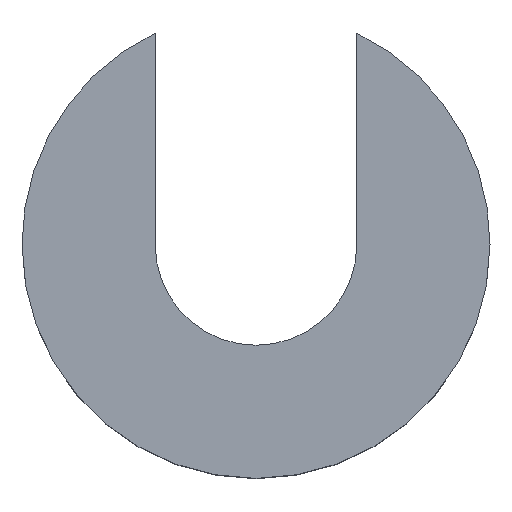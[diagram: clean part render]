
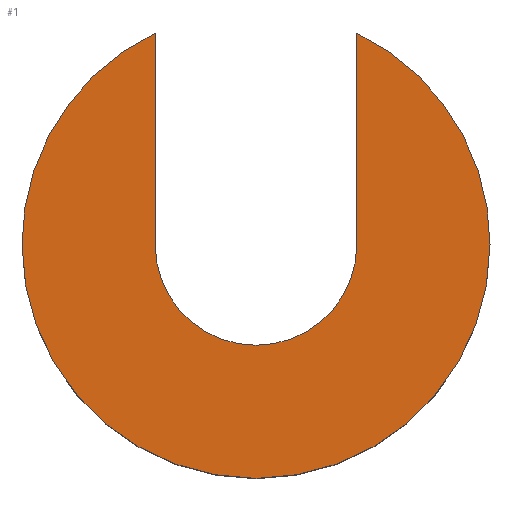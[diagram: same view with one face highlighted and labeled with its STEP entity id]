
A CAD part, top view. The second image highlights one B-rep face of the part: STEP entity #1.
In plain terms, the highlighted planar face has unit normal (0, 0, 1).
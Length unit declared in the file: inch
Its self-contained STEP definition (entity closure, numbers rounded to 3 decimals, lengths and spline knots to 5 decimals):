
#1 = ADVANCED_FACE ( 'NONE', ( #3 ), #357, .T. ) ;
#3 = FACE_OUTER_BOUND ( 'NONE', #412, .T. ) ;
#9 = DIRECTION ( 'NONE',  ( 1., 0., 0. ) ) ;
#15 = VECTOR ( 'NONE', #235, 39.37008 ) ;
#33 = CIRCLE ( 'NONE', #145, 0.725 ) ;
#46 = CARTESIAN_POINT ( 'NONE',  ( 0.3125, 0., 0.75 ) ) ;
#47 = CARTESIAN_POINT ( 'NONE',  ( -0.3125, 0., 0.75 ) ) ;
#73 = VECTOR ( 'NONE', #165, 39.37008 ) ;
#74 = EDGE_CURVE ( 'NONE', #184, #459, #276, .T. ) ;
#92 = EDGE_CURVE ( 'NONE', #459, #430, #388, .T. ) ;
#103 = DIRECTION ( 'NONE',  ( 0., 0., -1. ) ) ;
#118 = AXIS2_PLACEMENT_3D ( 'NONE', #179, #460, #325 ) ;
#119 = CARTESIAN_POINT ( 'NONE',  ( 0.725, 0., 0.75 ) ) ;
#123 = CIRCLE ( 'NONE', #170, 0.725 ) ;
#145 = AXIS2_PLACEMENT_3D ( 'NONE', #436, #271, #9 ) ;
#151 = EDGE_CURVE ( 'NONE', #400, #184, #166, .T. ) ;
#155 = CARTESIAN_POINT ( 'NONE',  ( 0., 0., 0.75 ) ) ;
#157 = CIRCLE ( 'NONE', #448, 0.725 ) ;
#165 = DIRECTION ( 'NONE',  ( 0., 1., 0. ) ) ;
#166 = LINE ( 'NONE', #201, #15 ) ;
#170 = AXIS2_PLACEMENT_3D ( 'NONE', #209, #349, #318 ) ;
#177 = EDGE_CURVE ( 'NONE', #368, #400, #33, .T. ) ;
#179 = CARTESIAN_POINT ( 'NONE',  ( 0., 0., 0.75 ) ) ;
#184 = VERTEX_POINT ( 'NONE', #46 ) ;
#201 = CARTESIAN_POINT ( 'NONE',  ( 0.3125, 0.65419, 0.75 ) ) ;
#204 = CARTESIAN_POINT ( 'NONE',  ( -0.3125, 0., 0.75 ) ) ;
#206 = EDGE_CURVE ( 'NONE', #430, #290, #123, .T. ) ;
#209 = CARTESIAN_POINT ( 'NONE',  ( 0., 0., 0.75 ) ) ;
#235 = DIRECTION ( 'NONE',  ( 0., -1., 0. ) ) ;
#237 = CARTESIAN_POINT ( 'NONE',  ( -0.3125, 0.65419, 0.75 ) ) ;
#271 = DIRECTION ( 'NONE',  ( 0., 0., 1. ) ) ;
#274 = ORIENTED_EDGE ( 'NONE', *, *, #151, .T. ) ;
#276 = CIRCLE ( 'NONE', #337, 0.3125 ) ;
#287 = DIRECTION ( 'NONE',  ( 1., 0., 0. ) ) ;
#290 = VERTEX_POINT ( 'NONE', #418 ) ;
#318 = DIRECTION ( 'NONE',  ( 1., 0., 0. ) ) ;
#325 = DIRECTION ( 'NONE',  ( 1., 0., 0. ) ) ;
#329 = ORIENTED_EDGE ( 'NONE', *, *, #177, .T. ) ;
#337 = AXIS2_PLACEMENT_3D ( 'NONE', #422, #103, #287 ) ;
#349 = DIRECTION ( 'NONE',  ( 0., 0., 1. ) ) ;
#357 = PLANE ( 'NONE',  #118 ) ;
#365 = ORIENTED_EDGE ( 'NONE', *, *, #369, .T. ) ;
#368 = VERTEX_POINT ( 'NONE', #119 ) ;
#369 = EDGE_CURVE ( 'NONE', #290, #368, #157, .T. ) ;
#378 = CARTESIAN_POINT ( 'NONE',  ( 0.3125, 0.65419, 0.75 ) ) ;
#388 = LINE ( 'NONE', #204, #73 ) ;
#395 = ORIENTED_EDGE ( 'NONE', *, *, #92, .T. ) ;
#400 = VERTEX_POINT ( 'NONE', #378 ) ;
#403 = DIRECTION ( 'NONE',  ( 0., 0., 1. ) ) ;
#411 = ORIENTED_EDGE ( 'NONE', *, *, #206, .T. ) ;
#412 = EDGE_LOOP ( 'NONE', ( #411, #365, #329, #274, #453, #395 ) ) ;
#418 = CARTESIAN_POINT ( 'NONE',  ( -0.725, 0., 0.75 ) ) ;
#422 = CARTESIAN_POINT ( 'NONE',  ( 0., 0., 0.75 ) ) ;
#430 = VERTEX_POINT ( 'NONE', #237 ) ;
#436 = CARTESIAN_POINT ( 'NONE',  ( 0., 0., 0.75 ) ) ;
#437 = DIRECTION ( 'NONE',  ( 1., 0., 0. ) ) ;
#448 = AXIS2_PLACEMENT_3D ( 'NONE', #155, #403, #437 ) ;
#453 = ORIENTED_EDGE ( 'NONE', *, *, #74, .T. ) ;
#459 = VERTEX_POINT ( 'NONE', #47 ) ;
#460 = DIRECTION ( 'NONE',  ( 0., 0., 1. ) ) ;
